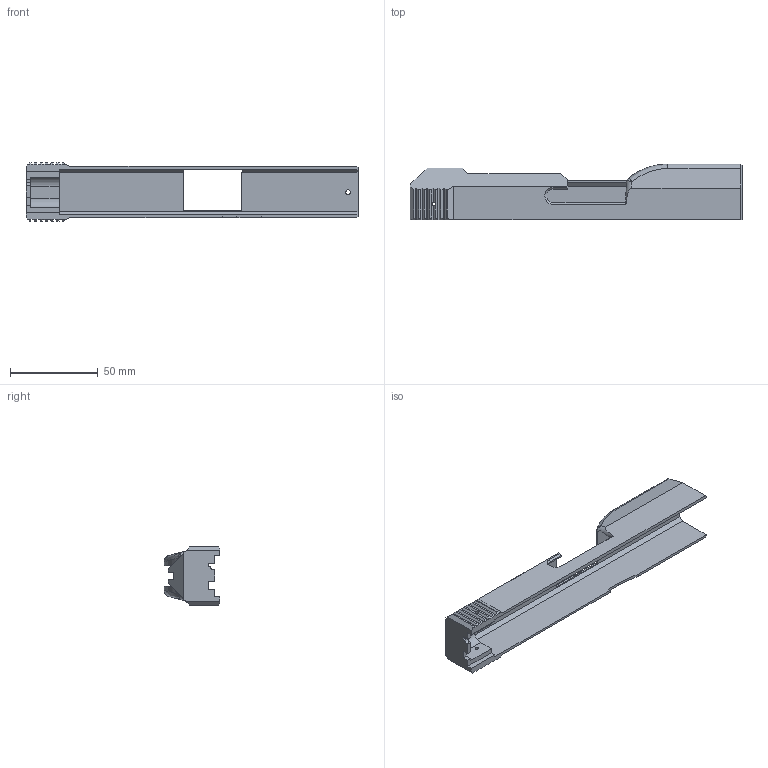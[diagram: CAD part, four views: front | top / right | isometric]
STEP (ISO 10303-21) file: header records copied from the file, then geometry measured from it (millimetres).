
FILE_DESCRIPTION(/* description */ (''),/* implementation_level */ '2;1');
FILE_NAME(/* name */ 'Halo Magnum Slide Cover.step',/* time_stamp */ '2022-03-30T10:09:04-06:00',/* author */ (''),/* organization */ (''),/* preprocessor_version */ 'ST-DEVELOPER v18.1',/* originating_system */ 'Autodesk Translation Framework v10.14.0.1471',/* authorisation */ '');
FILE_SCHEMA (('AUTOMOTIVE_DESIGN { 1 0 10303 214 3 1 1 }'));
Length unit declared in the file: millimetre
Products named in the file (1): Halo Magnum Beta
Bounding box: 189.39 x 31.84 x 33.19 mm (x, y, z)
Volume: 39591.8 mm3; surface area: 27736.4 mm2
Topology: 1 solids, 1 shells, 178 faces, 497 edges, 318 vertices
Faces by surface type: plane 156, cylinder 16, cone 4, bspline 2
Full cylindrical faces by diameter (mm): 2 x2, 2.7 x1
Entity records: 5712 total; most frequent: CARTESIAN_POINT 1042, ORIENTED_EDGE 994, DIRECTION 910, EDGE_CURVE 497, LINE 438, VECTOR 438, VERTEX_POINT 318, AXIS2_PLACEMENT_3D 236
